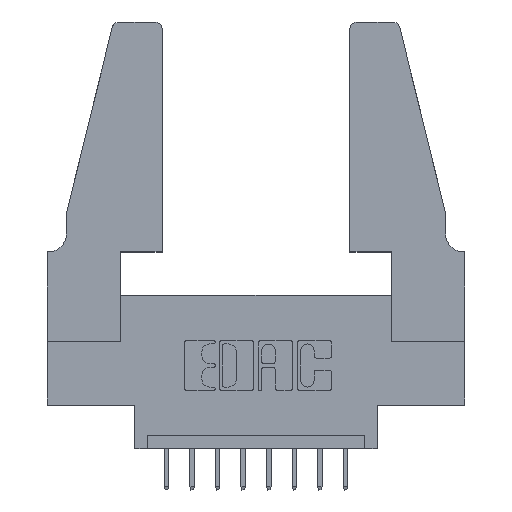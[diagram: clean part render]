
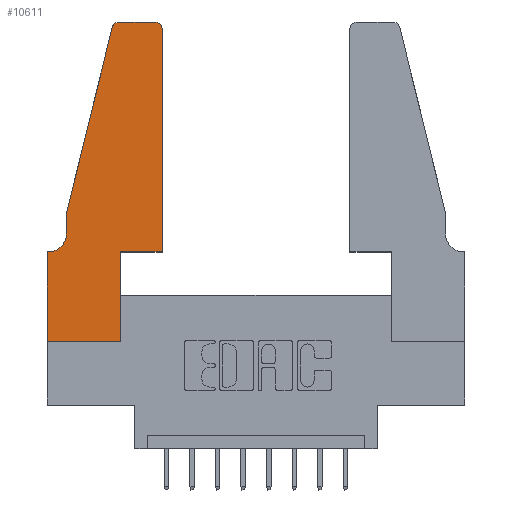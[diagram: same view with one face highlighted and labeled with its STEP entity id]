
A CAD part, top view. The second image highlights one B-rep face of the part: STEP entity #10611.
In plain terms, the highlighted planar face has unit normal (0, 0, 1).
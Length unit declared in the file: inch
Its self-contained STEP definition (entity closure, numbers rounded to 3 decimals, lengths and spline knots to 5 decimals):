
#140 = ORIENTED_EDGE ( 'NONE', *, *, #4843, .T. ) ;
#325 = EDGE_CURVE ( 'NONE', #3400, #8360, #5961, .T. ) ;
#360 = LINE ( 'NONE', #7348, #3485 ) ;
#371 = VECTOR ( 'NONE', #3469, 39.37008 ) ;
#403 = CARTESIAN_POINT ( 'NONE',  ( 0., 0., 0.37 ) ) ;
#423 = ORIENTED_EDGE ( 'NONE', *, *, #6572, .T. ) ;
#434 = DIRECTION ( 'NONE',  ( 0., 1., 0. ) ) ;
#445 = CARTESIAN_POINT ( 'NONE',  ( 0.4205, 1.25, 0.37 ) ) ;
#609 = LINE ( 'NONE', #9333, #3432 ) ;
#954 = VERTEX_POINT ( 'NONE', #5980 ) ;
#1037 = EDGE_CURVE ( 'NONE', #954, #4084, #8313, .T. ) ;
#1088 = DIRECTION ( 'NONE',  ( 0., 0., 1. ) ) ;
#1156 = LINE ( 'NONE', #7827, #3673 ) ;
#1394 = CARTESIAN_POINT ( 'NONE',  ( 0.4505, 1.22, 0.37 ) ) ;
#1403 = DIRECTION ( 'NONE',  ( 0., -1., 0. ) ) ;
#1437 = DIRECTION ( 'NONE',  ( 0., 0., -1. ) ) ;
#1502 = AXIS2_PLACEMENT_3D ( 'NONE', #8463, #1437, #12337 ) ;
#1553 = DIRECTION ( 'NONE',  ( 1., 0., 0. ) ) ;
#1642 = CARTESIAN_POINT ( 'NONE',  ( 0.4505, 0.35, 0.37 ) ) ;
#1830 = DIRECTION ( 'NONE',  ( 0., -1., 0. ) ) ;
#2103 = LINE ( 'NONE', #11146, #12109 ) ;
#2118 = DIRECTION ( 'NONE',  ( 1., 0., 0. ) ) ;
#2268 = LINE ( 'NONE', #11626, #371 ) ;
#2546 = ORIENTED_EDGE ( 'NONE', *, *, #9857, .T. ) ;
#2667 = CARTESIAN_POINT ( 'NONE',  ( 0.0755, 0.5, 0.37 ) ) ;
#3400 = VERTEX_POINT ( 'NONE', #7300 ) ;
#3432 = VECTOR ( 'NONE', #3477, 39.37008 ) ;
#3440 = CARTESIAN_POINT ( 'NONE',  ( 0.0055, 0.35, 0.37 ) ) ;
#3469 = DIRECTION ( 'NONE',  ( 0., 1., 0. ) ) ;
#3477 = DIRECTION ( 'NONE',  ( -0.239, -0.971, 0. ) ) ;
#3485 = VECTOR ( 'NONE', #434, 39.37008 ) ;
#3642 = VERTEX_POINT ( 'NONE', #8339 ) ;
#3668 = CARTESIAN_POINT ( 'NONE',  ( 0.0755, 0.42, 0.37 ) ) ;
#3673 = VECTOR ( 'NONE', #1830, 39.37008 ) ;
#3780 = ORIENTED_EDGE ( 'NONE', *, *, #4315, .T. ) ;
#3828 = AXIS2_PLACEMENT_3D ( 'NONE', #7614, #4633, #8725 ) ;
#3876 = CARTESIAN_POINT ( 'NONE',  ( 0.4505, 0.35, 0.37 ) ) ;
#4084 = VERTEX_POINT ( 'NONE', #3876 ) ;
#4095 = ORIENTED_EDGE ( 'NONE', *, *, #9729, .T. ) ;
#4154 = EDGE_CURVE ( 'NONE', #5793, #6307, #9178, .T. ) ;
#4315 = EDGE_CURVE ( 'NONE', #4084, #4812, #2268, .T. ) ;
#4548 = LINE ( 'NONE', #5536, #8172 ) ;
#4633 = DIRECTION ( 'NONE',  ( 0., 0., 1. ) ) ;
#4696 = DIRECTION ( 'NONE',  ( 1., 0., 0. ) ) ;
#4782 = CARTESIAN_POINT ( 'NONE',  ( 0., 0.35, 0.37 ) ) ;
#4812 = VERTEX_POINT ( 'NONE', #1394 ) ;
#4843 = EDGE_CURVE ( 'NONE', #3642, #954, #360, .T. ) ;
#5167 = EDGE_CURVE ( 'NONE', #6913, #3400, #12237, .T. ) ;
#5187 = EDGE_CURVE ( 'NONE', #6307, #7721, #9633, .T. ) ;
#5309 = DIRECTION ( 'NONE',  ( -1., 0., 0. ) ) ;
#5536 = CARTESIAN_POINT ( 'NONE',  ( 0., 0., 0.37 ) ) ;
#5793 = VERTEX_POINT ( 'NONE', #3668 ) ;
#5961 = CIRCLE ( 'NONE', #3828, 0.03 ) ;
#5980 = CARTESIAN_POINT ( 'NONE',  ( 0.2865, 0.35, 0.37 ) ) ;
#6307 = VERTEX_POINT ( 'NONE', #3440 ) ;
#6324 = FACE_OUTER_BOUND ( 'NONE', #8770, .T. ) ;
#6336 = DIRECTION ( 'NONE',  ( -1., 0., 0. ) ) ;
#6572 = EDGE_CURVE ( 'NONE', #4812, #6913, #9433, .T. ) ;
#6798 = EDGE_CURVE ( 'NONE', #8360, #8993, #609, .T. ) ;
#6913 = VERTEX_POINT ( 'NONE', #445 ) ;
#6924 = ORIENTED_EDGE ( 'NONE', *, *, #6946, .T. ) ;
#6946 = EDGE_CURVE ( 'NONE', #8722, #3642, #4548, .T. ) ;
#7300 = CARTESIAN_POINT ( 'NONE',  ( 0.284, 1.25, 0.37 ) ) ;
#7348 = CARTESIAN_POINT ( 'NONE',  ( 0.2865, 0.35, 0.37 ) ) ;
#7563 = VECTOR ( 'NONE', #5309, 39.37008 ) ;
#7580 = ORIENTED_EDGE ( 'NONE', *, *, #5167, .T. ) ;
#7614 = CARTESIAN_POINT ( 'NONE',  ( 0.284, 1.22, 0.37 ) ) ;
#7721 = VERTEX_POINT ( 'NONE', #4782 ) ;
#7827 = CARTESIAN_POINT ( 'NONE',  ( 0.0755, 0.5, 0.37 ) ) ;
#8154 = VECTOR ( 'NONE', #4696, 39.37008 ) ;
#8172 = VECTOR ( 'NONE', #1553, 39.37008 ) ;
#8313 = LINE ( 'NONE', #1642, #8154 ) ;
#8339 = CARTESIAN_POINT ( 'NONE',  ( 0.2865, 0., 0.37 ) ) ;
#8360 = VERTEX_POINT ( 'NONE', #12802 ) ;
#8463 = CARTESIAN_POINT ( 'NONE',  ( 0.0055, 0.42, 0.37 ) ) ;
#8486 = ORIENTED_EDGE ( 'NONE', *, *, #6798, .T. ) ;
#8722 = VERTEX_POINT ( 'NONE', #403 ) ;
#8725 = DIRECTION ( 'NONE',  ( 1., 0., 0. ) ) ;
#8770 = EDGE_LOOP ( 'NONE', ( #7580, #12265, #8486, #4095, #9699, #10733, #2546, #6924, #140, #8829, #3780, #423 ) ) ;
#8829 = ORIENTED_EDGE ( 'NONE', *, *, #1037, .T. ) ;
#8993 = VERTEX_POINT ( 'NONE', #2667 ) ;
#9022 = DIRECTION ( 'NONE',  ( 0., 0., 1. ) ) ;
#9109 = PLANE ( 'NONE',  #12952 ) ;
#9178 = CIRCLE ( 'NONE', #1502, 0.07 ) ;
#9333 = CARTESIAN_POINT ( 'NONE',  ( 0.0755, 0.5, 0.37 ) ) ;
#9433 = CIRCLE ( 'NONE', #11031, 0.03 ) ;
#9633 = LINE ( 'NONE', #10318, #11336 ) ;
#9699 = ORIENTED_EDGE ( 'NONE', *, *, #4154, .T. ) ;
#9729 = EDGE_CURVE ( 'NONE', #8993, #5793, #1156, .T. ) ;
#9857 = EDGE_CURVE ( 'NONE', #7721, #8722, #2103, .T. ) ;
#9990 = CARTESIAN_POINT ( 'NONE',  ( 0., 0.35, 0.37 ) ) ;
#10318 = CARTESIAN_POINT ( 'NONE',  ( 0.0755, 0.35, 0.37 ) ) ;
#10611 = ADVANCED_FACE ( 'NONE', ( #6324 ), #9109, .T. ) ;
#10733 = ORIENTED_EDGE ( 'NONE', *, *, #5187, .T. ) ;
#11013 = CARTESIAN_POINT ( 'NONE',  ( 0.4205, 1.22, 0.37 ) ) ;
#11031 = AXIS2_PLACEMENT_3D ( 'NONE', #11013, #1088, #2118 ) ;
#11146 = CARTESIAN_POINT ( 'NONE',  ( 0., 0., 0.37 ) ) ;
#11336 = VECTOR ( 'NONE', #6336, 39.37008 ) ;
#11626 = CARTESIAN_POINT ( 'NONE',  ( 0.4505, 0.35, 0.37 ) ) ;
#12109 = VECTOR ( 'NONE', #1403, 39.37008 ) ;
#12208 = CARTESIAN_POINT ( 'NONE',  ( 0.2605, 1.25, 0.37 ) ) ;
#12237 = LINE ( 'NONE', #12208, #7563 ) ;
#12265 = ORIENTED_EDGE ( 'NONE', *, *, #325, .T. ) ;
#12337 = DIRECTION ( 'NONE',  ( -1., 0., 0. ) ) ;
#12802 = CARTESIAN_POINT ( 'NONE',  ( 0.25487, 1.22718, 0.37 ) ) ;
#12932 = DIRECTION ( 'NONE',  ( 1., 0., 0. ) ) ;
#12952 = AXIS2_PLACEMENT_3D ( 'NONE', #9990, #9022, #12932 ) ;
